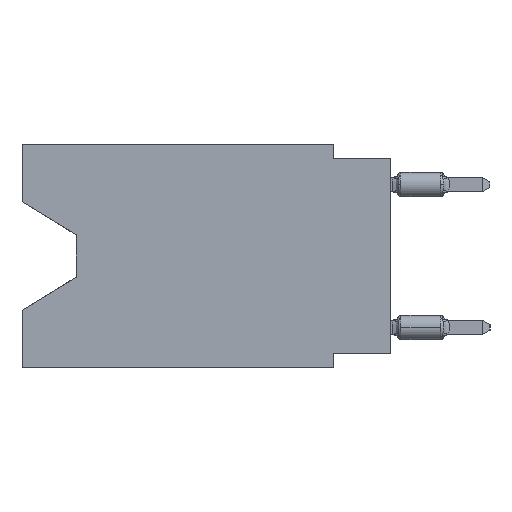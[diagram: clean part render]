
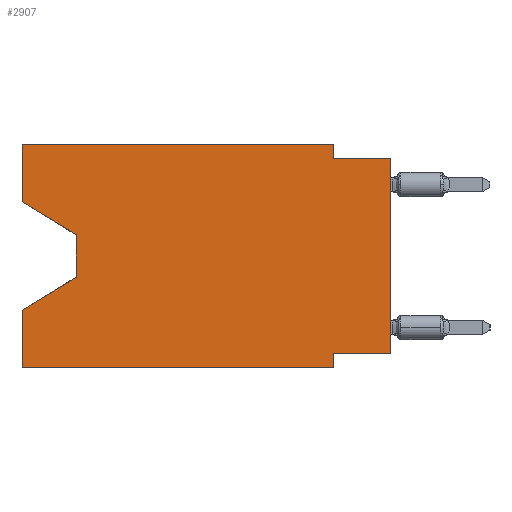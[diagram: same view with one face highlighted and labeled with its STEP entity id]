
A CAD part, left-side view. The second image highlights one B-rep face of the part: STEP entity #2907.
In plain terms, the highlighted planar face has unit normal (-1, 0, 0).
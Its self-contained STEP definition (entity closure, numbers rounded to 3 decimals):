
#7 = VECTOR ( 'NONE', #11269, 1000. ) ;
#268 = LINE ( 'NONE', #39507, #24978 ) ;
#752 = CARTESIAN_POINT ( 'NONE',  ( 0., 13.97, -5.893 ) ) ;
#1069 = CARTESIAN_POINT ( 'NONE',  ( 0., 0., -0.635 ) ) ;
#1269 = AXIS2_PLACEMENT_3D ( 'NONE', #26355, #36697, #6738 ) ;
#1713 = CARTESIAN_POINT ( 'NONE',  ( 0., 0., -9.271 ) ) ;
#1764 = VERTEX_POINT ( 'NONE', #21119 ) ;
#1959 = CARTESIAN_POINT ( 'NONE',  ( 0., 2.54, -9.271 ) ) ;
#2336 = DIRECTION ( 'NONE',  ( 0., 1., 0. ) ) ;
#2383 = LINE ( 'NONE', #15528, #10566 ) ;
#2657 = EDGE_LOOP ( 'NONE', ( #40671, #26053, #4766, #6043, #31933, #21213, #24134, #8055, #8327, #14586, #28900, #8584 ) ) ;
#2907 = ADVANCED_FACE ( 'NONE', ( #26780 ), #39083, .F. ) ;
#3447 = CARTESIAN_POINT ( 'NONE',  ( 0., 13.97, -4.013 ) ) ;
#3873 = LINE ( 'NONE', #3447, #39561 ) ;
#4386 = CARTESIAN_POINT ( 'NONE',  ( 0., 0., 0. ) ) ;
#4766 = ORIENTED_EDGE ( 'NONE', *, *, #38275, .T. ) ;
#5007 = CARTESIAN_POINT ( 'NONE',  ( 0., 0., -0.635 ) ) ;
#5832 = EDGE_CURVE ( 'NONE', #22848, #25293, #17868, .T. ) ;
#6043 = ORIENTED_EDGE ( 'NONE', *, *, #38039, .F. ) ;
#6738 = DIRECTION ( 'NONE',  ( 0., 0., -1. ) ) ;
#7574 = DIRECTION ( 'NONE',  ( 0., 0., 1. ) ) ;
#7731 = DIRECTION ( 'NONE',  ( 0., -1., 0. ) ) ;
#8055 = ORIENTED_EDGE ( 'NONE', *, *, #16568, .T. ) ;
#8327 = ORIENTED_EDGE ( 'NONE', *, *, #30555, .F. ) ;
#8584 = ORIENTED_EDGE ( 'NONE', *, *, #21962, .F. ) ;
#9377 = LINE ( 'NONE', #26422, #12760 ) ;
#10178 = VERTEX_POINT ( 'NONE', #29546 ) ;
#10482 = CARTESIAN_POINT ( 'NONE',  ( 0., 0., -9.271 ) ) ;
#10566 = VECTOR ( 'NONE', #42267, 1000. ) ;
#11248 = DIRECTION ( 'NONE',  ( 0., 0., -1. ) ) ;
#11269 = DIRECTION ( 'NONE',  ( 0., 0., 1. ) ) ;
#11301 = VECTOR ( 'NONE', #26199, 1000. ) ;
#12760 = VECTOR ( 'NONE', #22732, 1000. ) ;
#12819 = LINE ( 'NONE', #15827, #11301 ) ;
#13366 = CARTESIAN_POINT ( 'NONE',  ( 0., 13.97, -5.893 ) ) ;
#13657 = VERTEX_POINT ( 'NONE', #22035 ) ;
#13870 = EDGE_CURVE ( 'NONE', #25293, #13657, #23977, .T. ) ;
#14586 = ORIENTED_EDGE ( 'NONE', *, *, #32971, .F. ) ;
#14593 = VECTOR ( 'NONE', #16588, 1000. ) ;
#15137 = LINE ( 'NONE', #28507, #31910 ) ;
#15528 = CARTESIAN_POINT ( 'NONE',  ( 0., 16.383, 0. ) ) ;
#15827 = CARTESIAN_POINT ( 'NONE',  ( 0., 16.383, -2.546 ) ) ;
#16568 = EDGE_CURVE ( 'NONE', #22848, #20529, #20755, .T. ) ;
#16588 = DIRECTION ( 'NONE',  ( 0., 0.855, -0.519 ) ) ;
#16864 = LINE ( 'NONE', #20525, #39326 ) ;
#17868 = LINE ( 'NONE', #1713, #20902 ) ;
#19366 = DIRECTION ( 'NONE',  ( 0., 0., -1. ) ) ;
#19756 = CARTESIAN_POINT ( 'NONE',  ( 0., 13.97, -4.013 ) ) ;
#20525 = CARTESIAN_POINT ( 'NONE',  ( 0., 2.54, 0. ) ) ;
#20529 = VERTEX_POINT ( 'NONE', #5007 ) ;
#20755 = LINE ( 'NONE', #4386, #7 ) ;
#20818 = VERTEX_POINT ( 'NONE', #29791 ) ;
#20902 = VECTOR ( 'NONE', #2336, 1000. ) ;
#21086 = LINE ( 'NONE', #1069, #25808 ) ;
#21119 = CARTESIAN_POINT ( 'NONE',  ( 0., 2.54, -0.635 ) ) ;
#21213 = ORIENTED_EDGE ( 'NONE', *, *, #13870, .F. ) ;
#21389 = EDGE_CURVE ( 'NONE', #35250, #22827, #12819, .T. ) ;
#21839 = VECTOR ( 'NONE', #33903, 1000. ) ;
#21962 = EDGE_CURVE ( 'NONE', #35250, #20818, #268, .T. ) ;
#22035 = CARTESIAN_POINT ( 'NONE',  ( 0., 2.54, -9.906 ) ) ;
#22732 = DIRECTION ( 'NONE',  ( 0., -1., 0. ) ) ;
#22827 = VERTEX_POINT ( 'NONE', #19756 ) ;
#22848 = VERTEX_POINT ( 'NONE', #10482 ) ;
#23647 = EDGE_CURVE ( 'NONE', #27370, #13657, #15137, .T. ) ;
#23737 = CARTESIAN_POINT ( 'NONE',  ( 0., 16.383, -7.36 ) ) ;
#23943 = VERTEX_POINT ( 'NONE', #23737 ) ;
#23977 = LINE ( 'NONE', #34324, #21839 ) ;
#24134 = ORIENTED_EDGE ( 'NONE', *, *, #5832, .F. ) ;
#24978 = VECTOR ( 'NONE', #7574, 1000. ) ;
#25293 = VERTEX_POINT ( 'NONE', #1959 ) ;
#25808 = VECTOR ( 'NONE', #7731, 1000. ) ;
#26007 = CARTESIAN_POINT ( 'NONE',  ( 0., 16.383, -9.906 ) ) ;
#26053 = ORIENTED_EDGE ( 'NONE', *, *, #30324, .T. ) ;
#26199 = DIRECTION ( 'NONE',  ( 0., -0.855, -0.519 ) ) ;
#26355 = CARTESIAN_POINT ( 'NONE',  ( 0., 16.383, 0. ) ) ;
#26422 = CARTESIAN_POINT ( 'NONE',  ( 0., 16.383, 0. ) ) ;
#26780 = FACE_OUTER_BOUND ( 'NONE', #2657, .T. ) ;
#27370 = VERTEX_POINT ( 'NONE', #26007 ) ;
#28507 = CARTESIAN_POINT ( 'NONE',  ( 0., 16.383, -9.906 ) ) ;
#28900 = ORIENTED_EDGE ( 'NONE', *, *, #31191, .F. ) ;
#29546 = CARTESIAN_POINT ( 'NONE',  ( 0., 2.54, 0. ) ) ;
#29791 = CARTESIAN_POINT ( 'NONE',  ( 0., 16.383, 0. ) ) ;
#30324 = EDGE_CURVE ( 'NONE', #22827, #36200, #3873, .T. ) ;
#30555 = EDGE_CURVE ( 'NONE', #1764, #20529, #21086, .T. ) ;
#31191 = EDGE_CURVE ( 'NONE', #20818, #10178, #9377, .T. ) ;
#31910 = VECTOR ( 'NONE', #38626, 1000. ) ;
#31933 = ORIENTED_EDGE ( 'NONE', *, *, #23647, .T. ) ;
#32167 = CARTESIAN_POINT ( 'NONE',  ( 0., 16.383, -2.546 ) ) ;
#32971 = EDGE_CURVE ( 'NONE', #10178, #1764, #16864, .T. ) ;
#33903 = DIRECTION ( 'NONE',  ( 0., 0., -1. ) ) ;
#34324 = CARTESIAN_POINT ( 'NONE',  ( 0., 2.54, -9.906 ) ) ;
#35250 = VERTEX_POINT ( 'NONE', #32167 ) ;
#36010 = LINE ( 'NONE', #13366, #14593 ) ;
#36200 = VERTEX_POINT ( 'NONE', #752 ) ;
#36697 = DIRECTION ( 'NONE',  ( 1., 0., 0. ) ) ;
#38039 = EDGE_CURVE ( 'NONE', #27370, #23943, #2383, .T. ) ;
#38275 = EDGE_CURVE ( 'NONE', #36200, #23943, #36010, .T. ) ;
#38626 = DIRECTION ( 'NONE',  ( 0., -1., 0. ) ) ;
#39083 = PLANE ( 'NONE',  #1269 ) ;
#39326 = VECTOR ( 'NONE', #11248, 1000. ) ;
#39507 = CARTESIAN_POINT ( 'NONE',  ( 0., 16.383, 0. ) ) ;
#39561 = VECTOR ( 'NONE', #19366, 1000. ) ;
#40671 = ORIENTED_EDGE ( 'NONE', *, *, #21389, .T. ) ;
#42267 = DIRECTION ( 'NONE',  ( 0., 0., 1. ) ) ;
